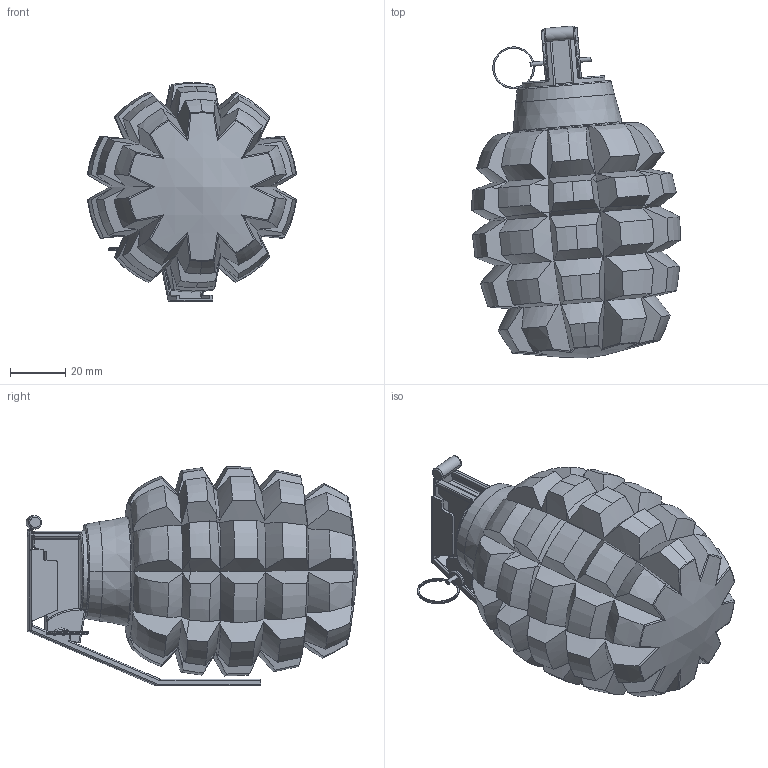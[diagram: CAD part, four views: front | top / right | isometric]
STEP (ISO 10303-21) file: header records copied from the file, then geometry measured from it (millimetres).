
FILE_DESCRIPTION (( 'STEP AP203' ), '1' );
FILE_NAME ('BombeD.STEP', '2012-09-02T04:48:47', ( 'Victor setia jaya' ), ( '' ), 'SwSTEP 2.0', 'SolidWorks 2012', '' );
FILE_SCHEMA (( 'CONFIG_CONTROL_DESIGN' ));
Length unit declared in the file: millimetre
Products named in the file (1): BombeD
Bounding box: 75.61 x 119.9 x 79.07 mm (x, y, z)
Volume: 284884 mm3; surface area: 40229.5 mm2
Topology: 1 solids, 1 shells, 477 faces, 1256 edges, 776 vertices
Faces by surface type: bspline 207, plane 99, cylinder 80, cone 41, torus 26, sphere 24
Entity records: 26938 total; most frequent: CARTESIAN_POINT 17115, ORIENTED_EDGE 2476, DIRECTION 1361, EDGE_CURVE 1238, VERTEX_POINT 767, B_SPLINE_CURVE_WITH_KNOTS 657, AXIS2_PLACEMENT_3D 529, EDGE_LOOP 481
